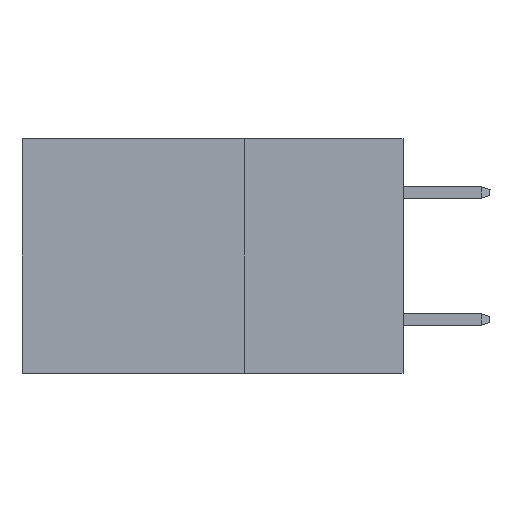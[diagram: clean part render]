
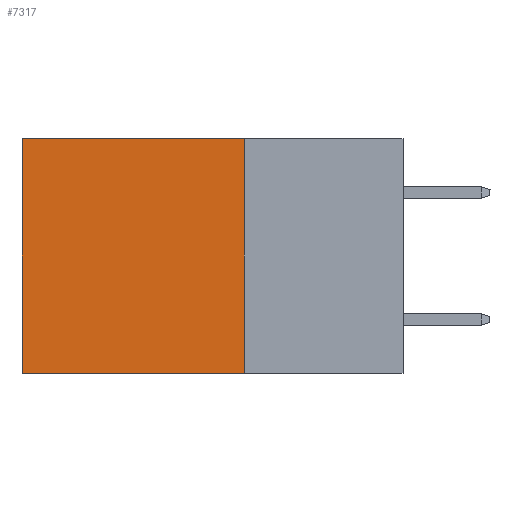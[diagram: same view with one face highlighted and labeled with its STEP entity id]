
A CAD part, left-side view. The second image highlights one B-rep face of the part: STEP entity #7317.
In plain terms, the highlighted planar face has unit normal (-1, 0, 0).
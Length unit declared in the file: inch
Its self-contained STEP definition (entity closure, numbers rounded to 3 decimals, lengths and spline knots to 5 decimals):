
#630 = EDGE_CURVE ( 'NONE', #12521, #2546, #10808, .T. ) ;
#1128 = LINE ( 'NONE', #10878, #4704 ) ;
#1135 = LINE ( 'NONE', #1245, #18751 ) ;
#1245 = CARTESIAN_POINT ( 'NONE',  ( 0.2875, 0.6, 0. ) ) ;
#1998 = AXIS2_PLACEMENT_3D ( 'NONE', #20600, #18771, #7567 ) ;
#2440 = ORIENTED_EDGE ( 'NONE', *, *, #17541, .F. ) ;
#2546 = VERTEX_POINT ( 'NONE', #8772 ) ;
#3198 = CARTESIAN_POINT ( 'NONE',  ( 0.2875, 0.6, 0. ) ) ;
#3248 = CARTESIAN_POINT ( 'NONE',  ( 0.2875, 0.25, -0.37 ) ) ;
#3680 = VERTEX_POINT ( 'NONE', #6624 ) ;
#4704 = VECTOR ( 'NONE', #5912, 39.37008 ) ;
#4744 = ORIENTED_EDGE ( 'NONE', *, *, #17412, .T. ) ;
#5448 = ORIENTED_EDGE ( 'NONE', *, *, #20291, .T. ) ;
#5912 = DIRECTION ( 'NONE',  ( 0., 1., 0. ) ) ;
#6624 = CARTESIAN_POINT ( 'NONE',  ( 0.2875, 0.25, 0. ) ) ;
#7317 = ADVANCED_FACE ( 'NONE', ( #20378 ), #12191, .F. ) ;
#7567 = DIRECTION ( 'NONE',  ( 0., 0., -1. ) ) ;
#8772 = CARTESIAN_POINT ( 'NONE',  ( 0.2875, 0.6, -0.37 ) ) ;
#9460 = LINE ( 'NONE', #21028, #14643 ) ;
#10808 = LINE ( 'NONE', #20850, #15677 ) ;
#10832 = ORIENTED_EDGE ( 'NONE', *, *, #630, .F. ) ;
#10878 = CARTESIAN_POINT ( 'NONE',  ( 0.2875, 0.25, 0. ) ) ;
#12191 = PLANE ( 'NONE',  #1998 ) ;
#12521 = VERTEX_POINT ( 'NONE', #3248 ) ;
#14643 = VECTOR ( 'NONE', #14964, 39.37008 ) ;
#14767 = DIRECTION ( 'NONE',  ( 0., 0., -1. ) ) ;
#14964 = DIRECTION ( 'NONE',  ( 0., 0., -1. ) ) ;
#15677 = VECTOR ( 'NONE', #17411, 39.37008 ) ;
#16196 = VERTEX_POINT ( 'NONE', #3198 ) ;
#17411 = DIRECTION ( 'NONE',  ( 0., 1., 0. ) ) ;
#17412 = EDGE_CURVE ( 'NONE', #16196, #2546, #1135, .T. ) ;
#17541 = EDGE_CURVE ( 'NONE', #3680, #12521, #9460, .T. ) ;
#18751 = VECTOR ( 'NONE', #14767, 39.37008 ) ;
#18771 = DIRECTION ( 'NONE',  ( 1., 0., 0. ) ) ;
#20291 = EDGE_CURVE ( 'NONE', #3680, #16196, #1128, .T. ) ;
#20378 = FACE_OUTER_BOUND ( 'NONE', #20562, .T. ) ;
#20562 = EDGE_LOOP ( 'NONE', ( #4744, #10832, #2440, #5448 ) ) ;
#20600 = CARTESIAN_POINT ( 'NONE',  ( 0.2875, 0.25, 0. ) ) ;
#20850 = CARTESIAN_POINT ( 'NONE',  ( 0.2875, 0.25, -0.37 ) ) ;
#21028 = CARTESIAN_POINT ( 'NONE',  ( 0.2875, 0.25, 0. ) ) ;
